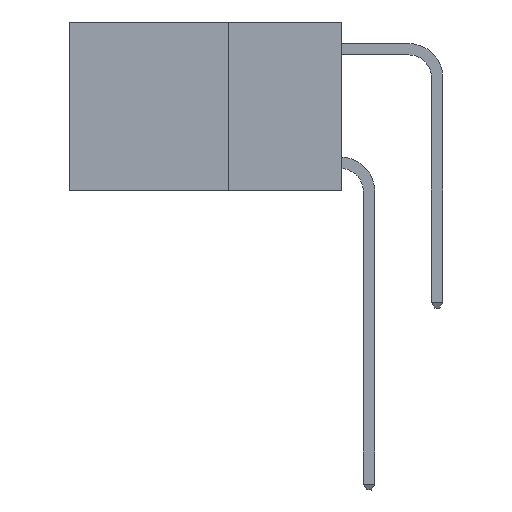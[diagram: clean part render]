
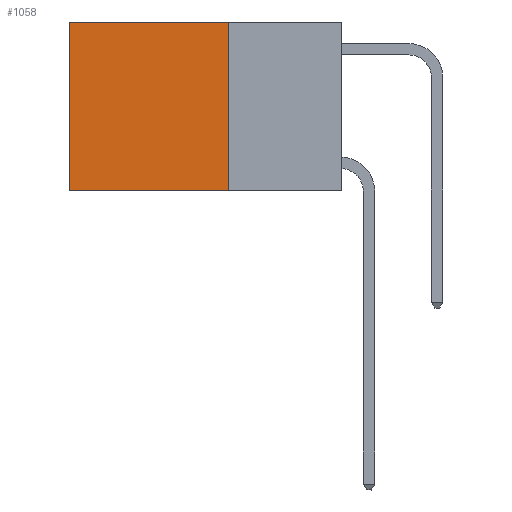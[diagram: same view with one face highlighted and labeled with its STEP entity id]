
A CAD part, left-side view. The second image highlights one B-rep face of the part: STEP entity #1058.
In plain terms, the highlighted planar face has unit normal (-1, 0, 0).
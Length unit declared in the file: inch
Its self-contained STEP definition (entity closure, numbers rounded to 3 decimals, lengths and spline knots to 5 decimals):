
#359 = VECTOR ( 'NONE', #1507, 39.37008 ) ;
#695 = LINE ( 'NONE', #7776, #359 ) ;
#1005 = VERTEX_POINT ( 'NONE', #9601 ) ;
#1058 = ADVANCED_FACE ( 'NONE', ( #11332 ), #6017, .F. ) ;
#1068 = VERTEX_POINT ( 'NONE', #5582 ) ;
#1397 = LINE ( 'NONE', #6704, #11936 ) ;
#1507 = DIRECTION ( 'NONE',  ( 0., 0., -1. ) ) ;
#1964 = VERTEX_POINT ( 'NONE', #8404 ) ;
#2647 = DIRECTION ( 'NONE',  ( 0., 0., -1. ) ) ;
#2919 = ORIENTED_EDGE ( 'NONE', *, *, #5635, .T. ) ;
#2924 = VERTEX_POINT ( 'NONE', #2991 ) ;
#2984 = ORIENTED_EDGE ( 'NONE', *, *, #8368, .F. ) ;
#2991 = CARTESIAN_POINT ( 'NONE',  ( 0.2625, 0.25, 0. ) ) ;
#3037 = ORIENTED_EDGE ( 'NONE', *, *, #10650, .F. ) ;
#3055 = ORIENTED_EDGE ( 'NONE', *, *, #9706, .T. ) ;
#4447 = EDGE_LOOP ( 'NONE', ( #2919, #2984, #3037, #3055 ) ) ;
#5360 = VECTOR ( 'NONE', #11880, 39.37008 ) ;
#5582 = CARTESIAN_POINT ( 'NONE',  ( 0.2625, 0.6, -0.37 ) ) ;
#5635 = EDGE_CURVE ( 'NONE', #1964, #1068, #695, .T. ) ;
#5959 = DIRECTION ( 'NONE',  ( 0., 0., -1. ) ) ;
#5987 = DIRECTION ( 'NONE',  ( 1., 0., 0. ) ) ;
#6017 = PLANE ( 'NONE',  #11971 ) ;
#6381 = CARTESIAN_POINT ( 'NONE',  ( 0.2625, 0.25, 0. ) ) ;
#6704 = CARTESIAN_POINT ( 'NONE',  ( 0.2625, 0.25, 0. ) ) ;
#7776 = CARTESIAN_POINT ( 'NONE',  ( 0.2625, 0.6, 0. ) ) ;
#7985 = LINE ( 'NONE', #8879, #5360 ) ;
#8368 = EDGE_CURVE ( 'NONE', #1005, #1068, #7985, .T. ) ;
#8404 = CARTESIAN_POINT ( 'NONE',  ( 0.2625, 0.6, 0. ) ) ;
#8484 = DIRECTION ( 'NONE',  ( 0., 1., 0. ) ) ;
#8879 = CARTESIAN_POINT ( 'NONE',  ( 0.2625, 0.25, -0.37 ) ) ;
#9601 = CARTESIAN_POINT ( 'NONE',  ( 0.2625, 0.25, -0.37 ) ) ;
#9706 = EDGE_CURVE ( 'NONE', #2924, #1964, #11037, .T. ) ;
#10441 = VECTOR ( 'NONE', #8484, 39.37008 ) ;
#10501 = CARTESIAN_POINT ( 'NONE',  ( 0.2625, 0.25, 0. ) ) ;
#10650 = EDGE_CURVE ( 'NONE', #2924, #1005, #1397, .T. ) ;
#11037 = LINE ( 'NONE', #10501, #10441 ) ;
#11332 = FACE_OUTER_BOUND ( 'NONE', #4447, .T. ) ;
#11880 = DIRECTION ( 'NONE',  ( 0., 1., 0. ) ) ;
#11936 = VECTOR ( 'NONE', #2647, 39.37008 ) ;
#11971 = AXIS2_PLACEMENT_3D ( 'NONE', #6381, #5987, #5959 ) ;
